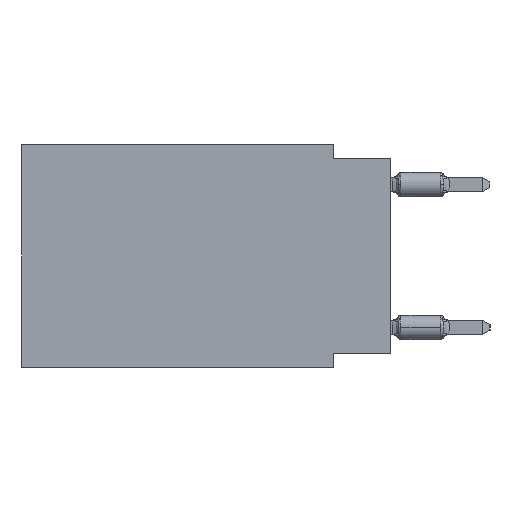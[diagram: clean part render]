
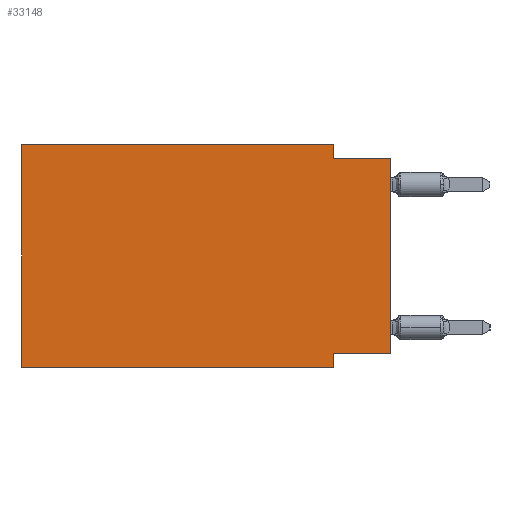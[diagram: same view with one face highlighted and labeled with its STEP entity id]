
A CAD part, left-side view. The second image highlights one B-rep face of the part: STEP entity #33148.
In plain terms, the highlighted planar face has unit normal (-1, 0, 0).
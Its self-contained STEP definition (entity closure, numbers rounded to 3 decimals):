
#354 = VECTOR ( 'NONE', #4906, 1000. ) ;
#1288 = DIRECTION ( 'NONE',  ( 0., 0., -1. ) ) ;
#1360 = VECTOR ( 'NONE', #59107, 1000. ) ;
#4657 = LINE ( 'NONE', #54360, #56960 ) ;
#4906 = DIRECTION ( 'NONE',  ( 0., 0., 1. ) ) ;
#4913 = EDGE_CURVE ( 'NONE', #35240, #62448, #57526, .T. ) ;
#5476 = CARTESIAN_POINT ( 'NONE',  ( 0., 16.383, -9.906 ) ) ;
#7796 = EDGE_LOOP ( 'NONE', ( #7999, #10276, #32728, #30529, #41520, #10467, #51293, #44838 ) ) ;
#7999 = ORIENTED_EDGE ( 'NONE', *, *, #51036, .T. ) ;
#10210 = VECTOR ( 'NONE', #14981, 1000. ) ;
#10276 = ORIENTED_EDGE ( 'NONE', *, *, #10800, .F. ) ;
#10467 = ORIENTED_EDGE ( 'NONE', *, *, #55781, .T. ) ;
#10659 = CARTESIAN_POINT ( 'NONE',  ( 0., 0., -0.635 ) ) ;
#10800 = EDGE_CURVE ( 'NONE', #45444, #52886, #51328, .T. ) ;
#11235 = LINE ( 'NONE', #30808, #59759 ) ;
#13724 = CARTESIAN_POINT ( 'NONE',  ( 0., 2.54, -9.906 ) ) ;
#14981 = DIRECTION ( 'NONE',  ( 0., 0., -1. ) ) ;
#15307 = DIRECTION ( 'NONE',  ( 0., -1., 0. ) ) ;
#19458 = DIRECTION ( 'NONE',  ( 0., 0., -1. ) ) ;
#23674 = LINE ( 'NONE', #13724, #10210 ) ;
#24622 = AXIS2_PLACEMENT_3D ( 'NONE', #33594, #58905, #19458 ) ;
#25671 = VERTEX_POINT ( 'NONE', #40243 ) ;
#27752 = VECTOR ( 'NONE', #57488, 1000. ) ;
#28719 = CARTESIAN_POINT ( 'NONE',  ( 0., 2.54, -0.635 ) ) ;
#29352 = DIRECTION ( 'NONE',  ( 0., 0., 1. ) ) ;
#30514 = CARTESIAN_POINT ( 'NONE',  ( 0., 0., -0.635 ) ) ;
#30529 = ORIENTED_EDGE ( 'NONE', *, *, #59040, .F. ) ;
#30808 = CARTESIAN_POINT ( 'NONE',  ( 0., 2.54, 0. ) ) ;
#31018 = LINE ( 'NONE', #45478, #41214 ) ;
#32728 = ORIENTED_EDGE ( 'NONE', *, *, #38251, .F. ) ;
#33148 = ADVANCED_FACE ( 'NONE', ( #39365 ), #43551, .F. ) ;
#33594 = CARTESIAN_POINT ( 'NONE',  ( 0., 16.383, 0. ) ) ;
#35240 = VERTEX_POINT ( 'NONE', #5476 ) ;
#36993 = CARTESIAN_POINT ( 'NONE',  ( 0., 16.383, -9.906 ) ) ;
#38144 = CARTESIAN_POINT ( 'NONE',  ( 0., 2.54, -9.906 ) ) ;
#38251 = EDGE_CURVE ( 'NONE', #41961, #45444, #11235, .T. ) ;
#39365 = FACE_OUTER_BOUND ( 'NONE', #7796, .T. ) ;
#39570 = CARTESIAN_POINT ( 'NONE',  ( 0., 0., -9.271 ) ) ;
#40243 = CARTESIAN_POINT ( 'NONE',  ( 0., 2.54, -9.271 ) ) ;
#41214 = VECTOR ( 'NONE', #15307, 1000. ) ;
#41302 = VECTOR ( 'NONE', #50070, 1000. ) ;
#41520 = ORIENTED_EDGE ( 'NONE', *, *, #4913, .F. ) ;
#41961 = VERTEX_POINT ( 'NONE', #52708 ) ;
#43495 = CARTESIAN_POINT ( 'NONE',  ( 0., 16.383, 0. ) ) ;
#43551 = PLANE ( 'NONE',  #24622 ) ;
#44838 = ORIENTED_EDGE ( 'NONE', *, *, #59997, .F. ) ;
#45444 = VERTEX_POINT ( 'NONE', #28719 ) ;
#45478 = CARTESIAN_POINT ( 'NONE',  ( 0., 16.383, 0. ) ) ;
#45906 = VERTEX_POINT ( 'NONE', #38144 ) ;
#48666 = VERTEX_POINT ( 'NONE', #56689 ) ;
#49178 = LINE ( 'NONE', #39570, #1360 ) ;
#50070 = DIRECTION ( 'NONE',  ( 0., -1., 0. ) ) ;
#51036 = EDGE_CURVE ( 'NONE', #48666, #52886, #4657, .T. ) ;
#51293 = ORIENTED_EDGE ( 'NONE', *, *, #63223, .F. ) ;
#51328 = LINE ( 'NONE', #30514, #41302 ) ;
#52708 = CARTESIAN_POINT ( 'NONE',  ( 0., 2.54, 0. ) ) ;
#52886 = VERTEX_POINT ( 'NONE', #10659 ) ;
#53021 = CARTESIAN_POINT ( 'NONE',  ( 0., 16.383, 0. ) ) ;
#54360 = CARTESIAN_POINT ( 'NONE',  ( 0., 0., 0. ) ) ;
#55781 = EDGE_CURVE ( 'NONE', #35240, #45906, #61348, .T. ) ;
#56689 = CARTESIAN_POINT ( 'NONE',  ( 0., 0., -9.271 ) ) ;
#56960 = VECTOR ( 'NONE', #29352, 1000. ) ;
#57488 = DIRECTION ( 'NONE',  ( 0., -1., 0. ) ) ;
#57526 = LINE ( 'NONE', #53021, #354 ) ;
#58905 = DIRECTION ( 'NONE',  ( 1., 0., 0. ) ) ;
#59040 = EDGE_CURVE ( 'NONE', #62448, #41961, #31018, .T. ) ;
#59107 = DIRECTION ( 'NONE',  ( 0., 1., 0. ) ) ;
#59759 = VECTOR ( 'NONE', #1288, 1000. ) ;
#59997 = EDGE_CURVE ( 'NONE', #48666, #25671, #49178, .T. ) ;
#61348 = LINE ( 'NONE', #36993, #27752 ) ;
#62448 = VERTEX_POINT ( 'NONE', #43495 ) ;
#63223 = EDGE_CURVE ( 'NONE', #25671, #45906, #23674, .T. ) ;
